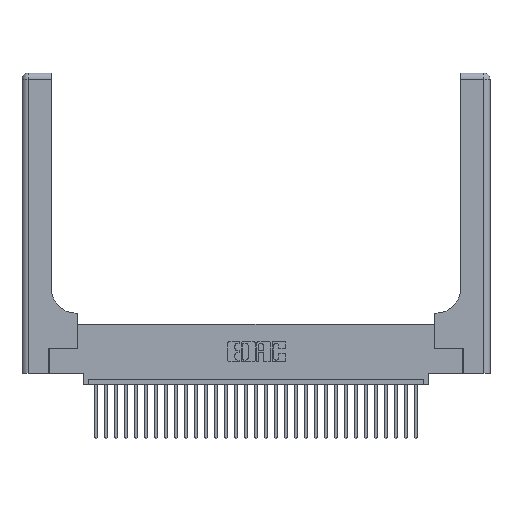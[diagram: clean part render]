
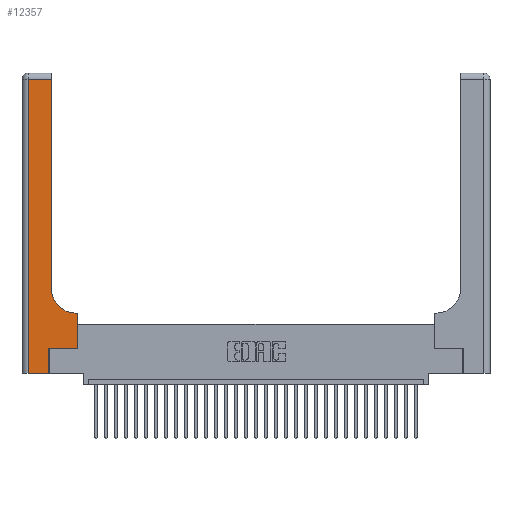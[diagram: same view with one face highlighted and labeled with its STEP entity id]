
A CAD part, top view. The second image highlights one B-rep face of the part: STEP entity #12357.
In plain terms, the highlighted planar face has unit normal (0, 0, 1).
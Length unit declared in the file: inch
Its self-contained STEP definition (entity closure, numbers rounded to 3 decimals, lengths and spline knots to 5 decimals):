
#529 = EDGE_CURVE ( 'NONE', #17726, #25666, #24770, .T. ) ;
#1858 = AXIS2_PLACEMENT_3D ( 'NONE', #17110, #21863, #29089 ) ;
#2024 = VERTEX_POINT ( 'NONE', #23173 ) ;
#2336 = VECTOR ( 'NONE', #10632, 39.37008 ) ;
#2542 = VECTOR ( 'NONE', #14335, 39.37008 ) ;
#2618 = CARTESIAN_POINT ( 'NONE',  ( 0.269, 0.25, 0.37 ) ) ;
#3037 = VECTOR ( 'NONE', #22112, 39.37008 ) ;
#3363 = CARTESIAN_POINT ( 'NONE',  ( 0.2915, 3., 0.37 ) ) ;
#3521 = CARTESIAN_POINT ( 'NONE',  ( 0.06, 2.94, 0.37 ) ) ;
#4554 = ORIENTED_EDGE ( 'NONE', *, *, #21898, .T. ) ;
#4914 = CARTESIAN_POINT ( 'NONE',  ( 0.06, 0., 0.37 ) ) ;
#6624 = ORIENTED_EDGE ( 'NONE', *, *, #24378, .T. ) ;
#7050 = CARTESIAN_POINT ( 'NONE',  ( 0.5415, 0.6, 0.37 ) ) ;
#7389 = CARTESIAN_POINT ( 'NONE',  ( 0., 0., 0.37 ) ) ;
#8097 = CARTESIAN_POINT ( 'NONE',  ( 0.2915, 0.85, 0.37 ) ) ;
#8396 = ORIENTED_EDGE ( 'NONE', *, *, #13656, .T. ) ;
#8617 = LINE ( 'NONE', #2618, #18129 ) ;
#9045 = DIRECTION ( 'NONE',  ( 0., 1., 0. ) ) ;
#9285 = EDGE_LOOP ( 'NONE', ( #6624, #8396, #17474, #4554, #10691, #16406, #20714, #17954, #18847 ) ) ;
#9612 = VERTEX_POINT ( 'NONE', #26235 ) ;
#10344 = LINE ( 'NONE', #29327, #26262 ) ;
#10632 = DIRECTION ( 'NONE',  ( -1., 0., 0. ) ) ;
#10659 = LINE ( 'NONE', #30170, #2336 ) ;
#10691 = ORIENTED_EDGE ( 'NONE', *, *, #12154, .T. ) ;
#11028 = EDGE_CURVE ( 'NONE', #2024, #30054, #8617, .T. ) ;
#12154 = EDGE_CURVE ( 'NONE', #18205, #2024, #13156, .T. ) ;
#12357 = ADVANCED_FACE ( 'NONE', ( #30608 ), #28258, .F. ) ;
#13156 = LINE ( 'NONE', #21768, #2542 ) ;
#13656 = EDGE_CURVE ( 'NONE', #9612, #17726, #10344, .T. ) ;
#14335 = DIRECTION ( 'NONE',  ( 0., 1., 0. ) ) ;
#15136 = DIRECTION ( 'NONE',  ( -1., 0., 0. ) ) ;
#15221 = EDGE_CURVE ( 'NONE', #27053, #27353, #10659, .T. ) ;
#16406 = ORIENTED_EDGE ( 'NONE', *, *, #11028, .T. ) ;
#16892 = VECTOR ( 'NONE', #27315, 39.37008 ) ;
#17110 = CARTESIAN_POINT ( 'NONE',  ( 0.5415, 0.85, 0.37 ) ) ;
#17372 = DIRECTION ( 'NONE',  ( 1., 0., 0. ) ) ;
#17474 = ORIENTED_EDGE ( 'NONE', *, *, #529, .T. ) ;
#17726 = VERTEX_POINT ( 'NONE', #3521 ) ;
#17954 = ORIENTED_EDGE ( 'NONE', *, *, #15221, .T. ) ;
#18129 = VECTOR ( 'NONE', #17372, 39.37008 ) ;
#18184 = LINE ( 'NONE', #26178, #31061 ) ;
#18205 = VERTEX_POINT ( 'NONE', #28560 ) ;
#18847 = ORIENTED_EDGE ( 'NONE', *, *, #25653, .T. ) ;
#20714 = ORIENTED_EDGE ( 'NONE', *, *, #22752, .T. ) ;
#20719 = AXIS2_PLACEMENT_3D ( 'NONE', #26013, #26207, #31013 ) ;
#21395 = VECTOR ( 'NONE', #28610, 39.37008 ) ;
#21768 = CARTESIAN_POINT ( 'NONE',  ( 0.269, 0., 0.37 ) ) ;
#21863 = DIRECTION ( 'NONE',  ( 0., 0., -1. ) ) ;
#21898 = EDGE_CURVE ( 'NONE', #25666, #18205, #26526, .T. ) ;
#22112 = DIRECTION ( 'NONE',  ( 1., 0., 0. ) ) ;
#22752 = EDGE_CURVE ( 'NONE', #30054, #27053, #18184, .T. ) ;
#23173 = CARTESIAN_POINT ( 'NONE',  ( 0.269, 0.25, 0.37 ) ) ;
#23307 = LINE ( 'NONE', #3363, #16892 ) ;
#23617 = CARTESIAN_POINT ( 'NONE',  ( 0.06, 3., 0.37 ) ) ;
#24378 = EDGE_CURVE ( 'NONE', #30118, #9612, #23307, .T. ) ;
#24770 = LINE ( 'NONE', #23617, #21395 ) ;
#25594 = CARTESIAN_POINT ( 'NONE',  ( 0.5585, 0.6, 0.37 ) ) ;
#25653 = EDGE_CURVE ( 'NONE', #27353, #30118, #30317, .T. ) ;
#25666 = VERTEX_POINT ( 'NONE', #4914 ) ;
#26013 = CARTESIAN_POINT ( 'NONE',  ( 0., 3., 0.37 ) ) ;
#26178 = CARTESIAN_POINT ( 'NONE',  ( 0.5585, 0.25, 0.37 ) ) ;
#26207 = DIRECTION ( 'NONE',  ( 0., 0., -1. ) ) ;
#26235 = CARTESIAN_POINT ( 'NONE',  ( 0.2915, 2.94, 0.37 ) ) ;
#26262 = VECTOR ( 'NONE', #15136, 39.37008 ) ;
#26526 = LINE ( 'NONE', #7389, #3037 ) ;
#27053 = VERTEX_POINT ( 'NONE', #25594 ) ;
#27288 = CARTESIAN_POINT ( 'NONE',  ( 0.5585, 0.25, 0.37 ) ) ;
#27315 = DIRECTION ( 'NONE',  ( 0., 1., 0. ) ) ;
#27353 = VERTEX_POINT ( 'NONE', #7050 ) ;
#28258 = PLANE ( 'NONE',  #20719 ) ;
#28560 = CARTESIAN_POINT ( 'NONE',  ( 0.269, 0., 0.37 ) ) ;
#28610 = DIRECTION ( 'NONE',  ( 0., -1., 0. ) ) ;
#29089 = DIRECTION ( 'NONE',  ( 1., 0., 0. ) ) ;
#29327 = CARTESIAN_POINT ( 'NONE',  ( 0., 2.94, 0.37 ) ) ;
#30054 = VERTEX_POINT ( 'NONE', #27288 ) ;
#30118 = VERTEX_POINT ( 'NONE', #8097 ) ;
#30170 = CARTESIAN_POINT ( 'NONE',  ( 0.2915, 0.6, 0.37 ) ) ;
#30317 = CIRCLE ( 'NONE', #1858, 0.25 ) ;
#30608 = FACE_OUTER_BOUND ( 'NONE', #9285, .T. ) ;
#31013 = DIRECTION ( 'NONE',  ( -1., 0., 0. ) ) ;
#31061 = VECTOR ( 'NONE', #9045, 39.37008 ) ;
